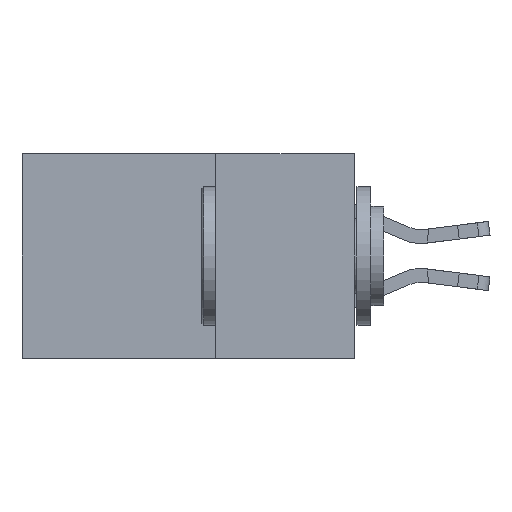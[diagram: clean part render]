
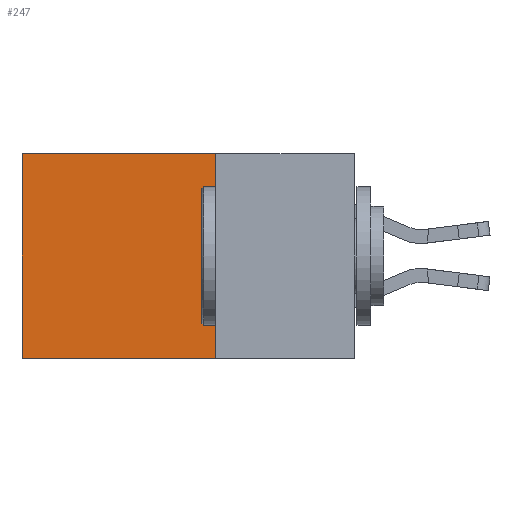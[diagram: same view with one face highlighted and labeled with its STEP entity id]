
A CAD part, left-side view. The second image highlights one B-rep face of the part: STEP entity #247.
In plain terms, the highlighted planar face has unit normal (-1, 0, 0).
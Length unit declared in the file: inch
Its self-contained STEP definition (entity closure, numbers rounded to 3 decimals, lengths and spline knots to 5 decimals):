
#247 = ADVANCED_FACE ( 'NONE', ( #312 ), #18835, .F. ) ;
#312 = FACE_OUTER_BOUND ( 'NONE', #1234, .T. ) ;
#646 = DIRECTION ( 'NONE',  ( 0., 0., -1. ) ) ;
#1097 = VECTOR ( 'NONE', #21512, 39.37008 ) ;
#1234 = EDGE_LOOP ( 'NONE', ( #11045, #16704, #9883, #15848 ) ) ;
#1464 = VECTOR ( 'NONE', #21528, 39.37008 ) ;
#1692 = LINE ( 'NONE', #14048, #21262 ) ;
#2504 = CARTESIAN_POINT ( 'NONE',  ( 0.298, 0.6, 0. ) ) ;
#2567 = CARTESIAN_POINT ( 'NONE',  ( 0.298, 0.25, 0. ) ) ;
#4816 = VERTEX_POINT ( 'NONE', #16029 ) ;
#5958 = AXIS2_PLACEMENT_3D ( 'NONE', #21127, #18773, #16061 ) ;
#6772 = EDGE_CURVE ( 'NONE', #12299, #13761, #1692, .T. ) ;
#7427 = LINE ( 'NONE', #13770, #20633 ) ;
#7977 = VERTEX_POINT ( 'NONE', #12894 ) ;
#9883 = ORIENTED_EDGE ( 'NONE', *, *, #6772, .F. ) ;
#11045 = ORIENTED_EDGE ( 'NONE', *, *, #18667, .T. ) ;
#11673 = EDGE_CURVE ( 'NONE', #13761, #7977, #7427, .T. ) ;
#12299 = VERTEX_POINT ( 'NONE', #21507 ) ;
#12894 = CARTESIAN_POINT ( 'NONE',  ( 0.298, 0.6, -0.37 ) ) ;
#13761 = VERTEX_POINT ( 'NONE', #23767 ) ;
#13770 = CARTESIAN_POINT ( 'NONE',  ( 0.298, 0.25, -0.37 ) ) ;
#14048 = CARTESIAN_POINT ( 'NONE',  ( 0.298, 0.25, 0. ) ) ;
#15330 = LINE ( 'NONE', #2504, #1464 ) ;
#15848 = ORIENTED_EDGE ( 'NONE', *, *, #16010, .T. ) ;
#16010 = EDGE_CURVE ( 'NONE', #12299, #4816, #16943, .T. ) ;
#16029 = CARTESIAN_POINT ( 'NONE',  ( 0.298, 0.6, 0. ) ) ;
#16061 = DIRECTION ( 'NONE',  ( 0., 0., -1. ) ) ;
#16704 = ORIENTED_EDGE ( 'NONE', *, *, #11673, .F. ) ;
#16943 = LINE ( 'NONE', #2567, #1097 ) ;
#18667 = EDGE_CURVE ( 'NONE', #4816, #7977, #15330, .T. ) ;
#18773 = DIRECTION ( 'NONE',  ( 1., 0., 0. ) ) ;
#18835 = PLANE ( 'NONE',  #5958 ) ;
#20633 = VECTOR ( 'NONE', #21285, 39.37008 ) ;
#21127 = CARTESIAN_POINT ( 'NONE',  ( 0.298, 0.25, 0. ) ) ;
#21262 = VECTOR ( 'NONE', #646, 39.37008 ) ;
#21285 = DIRECTION ( 'NONE',  ( 0., 1., 0. ) ) ;
#21507 = CARTESIAN_POINT ( 'NONE',  ( 0.298, 0.25, 0. ) ) ;
#21512 = DIRECTION ( 'NONE',  ( 0., 1., 0. ) ) ;
#21528 = DIRECTION ( 'NONE',  ( 0., 0., -1. ) ) ;
#23767 = CARTESIAN_POINT ( 'NONE',  ( 0.298, 0.25, -0.37 ) ) ;
